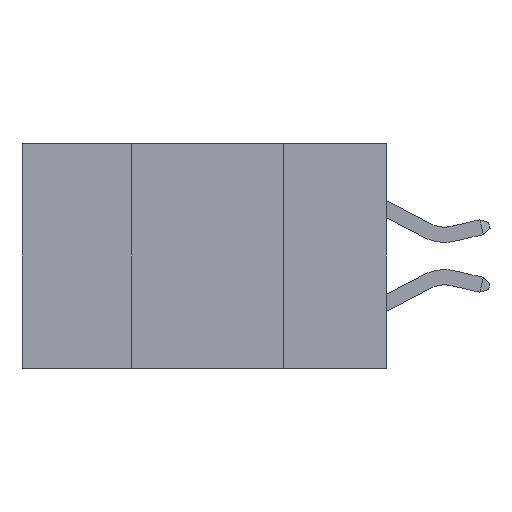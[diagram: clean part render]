
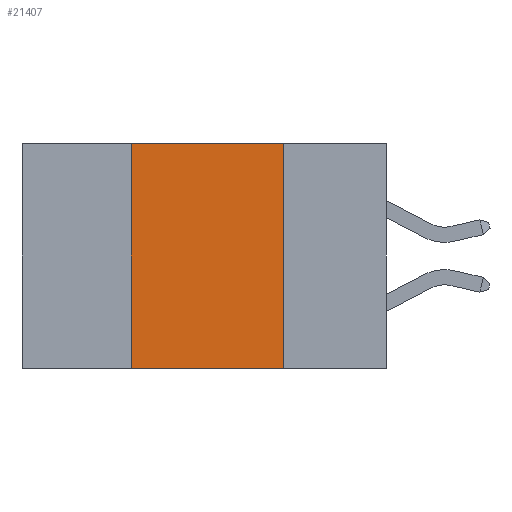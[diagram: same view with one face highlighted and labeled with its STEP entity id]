
A CAD part, left-side view. The second image highlights one B-rep face of the part: STEP entity #21407.
In plain terms, the highlighted planar face has unit normal (-1, 0, 0).
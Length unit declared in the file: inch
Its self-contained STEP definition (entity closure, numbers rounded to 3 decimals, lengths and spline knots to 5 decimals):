
#350 = EDGE_CURVE ( 'NONE', #18932, #19784, #11651, .T. ) ;
#977 = DIRECTION ( 'NONE',  ( 0., -1., 0. ) ) ;
#1273 = CARTESIAN_POINT ( 'NONE',  ( 0., 0.42, -0.37 ) ) ;
#1455 = FACE_OUTER_BOUND ( 'NONE', #9538, .T. ) ;
#2360 = DIRECTION ( 'NONE',  ( 0., 0., 1. ) ) ;
#2783 = CARTESIAN_POINT ( 'NONE',  ( 0., 0.17, -0.37 ) ) ;
#2848 = DIRECTION ( 'NONE',  ( 0., 0., -1. ) ) ;
#3330 = VECTOR ( 'NONE', #2848, 39.37008 ) ;
#3553 = LINE ( 'NONE', #13859, #17882 ) ;
#3692 = CARTESIAN_POINT ( 'NONE',  ( 0., 0.17, 0. ) ) ;
#3828 = ORIENTED_EDGE ( 'NONE', *, *, #22600, .F. ) ;
#4502 = DIRECTION ( 'NONE',  ( 1., 0., 0. ) ) ;
#4731 = PLANE ( 'NONE',  #5201 ) ;
#5201 = AXIS2_PLACEMENT_3D ( 'NONE', #8526, #4502, #11783 ) ;
#8526 = CARTESIAN_POINT ( 'NONE',  ( 0., 0.6, 0. ) ) ;
#9538 = EDGE_LOOP ( 'NONE', ( #3828, #16549, #11377, #17214 ) ) ;
#11377 = ORIENTED_EDGE ( 'NONE', *, *, #11794, .F. ) ;
#11490 = CARTESIAN_POINT ( 'NONE',  ( 0., 0.42, 0. ) ) ;
#11651 = LINE ( 'NONE', #18735, #19253 ) ;
#11783 = DIRECTION ( 'NONE',  ( 0., 0., -1. ) ) ;
#11794 = EDGE_CURVE ( 'NONE', #18194, #18932, #14863, .T. ) ;
#13859 = CARTESIAN_POINT ( 'NONE',  ( 0., 0.6, -0.37 ) ) ;
#13955 = DIRECTION ( 'NONE',  ( 0., -1., 0. ) ) ;
#13979 = EDGE_CURVE ( 'NONE', #18194, #16515, #3553, .T. ) ;
#14863 = LINE ( 'NONE', #16715, #19279 ) ;
#16515 = VERTEX_POINT ( 'NONE', #2783 ) ;
#16549 = ORIENTED_EDGE ( 'NONE', *, *, #350, .F. ) ;
#16715 = CARTESIAN_POINT ( 'NONE',  ( 0., 0.42, -0.37 ) ) ;
#16869 = CARTESIAN_POINT ( 'NONE',  ( 0., 0.17, -0.37 ) ) ;
#17214 = ORIENTED_EDGE ( 'NONE', *, *, #13979, .T. ) ;
#17882 = VECTOR ( 'NONE', #13955, 39.37008 ) ;
#18194 = VERTEX_POINT ( 'NONE', #1273 ) ;
#18735 = CARTESIAN_POINT ( 'NONE',  ( 0., 0.6, 0. ) ) ;
#18748 = LINE ( 'NONE', #16869, #3330 ) ;
#18932 = VERTEX_POINT ( 'NONE', #11490 ) ;
#19253 = VECTOR ( 'NONE', #977, 39.37008 ) ;
#19279 = VECTOR ( 'NONE', #2360, 39.37008 ) ;
#19784 = VERTEX_POINT ( 'NONE', #3692 ) ;
#21407 = ADVANCED_FACE ( 'NONE', ( #1455 ), #4731, .F. ) ;
#22600 = EDGE_CURVE ( 'NONE', #19784, #16515, #18748, .T. ) ;
